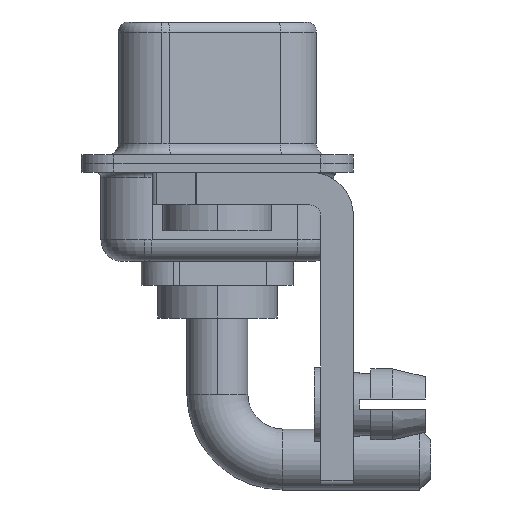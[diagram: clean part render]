
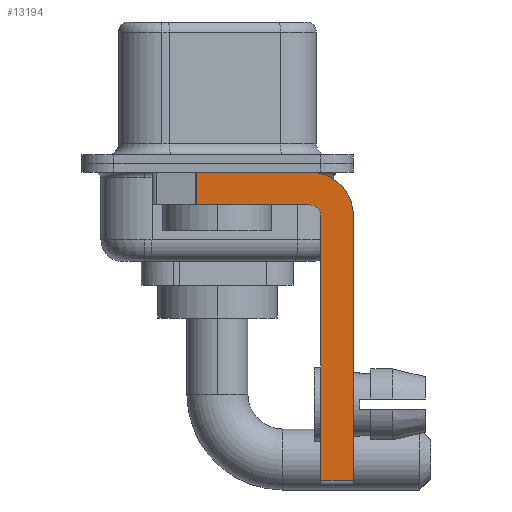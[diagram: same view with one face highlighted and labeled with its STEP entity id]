
A CAD part, left-side view. The second image highlights one B-rep face of the part: STEP entity #13194.
In plain terms, the highlighted planar face has unit normal (-1, 0, 0).
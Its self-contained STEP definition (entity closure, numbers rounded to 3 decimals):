
#27 = EDGE_CURVE ( 'NONE', #10403, #17854, #42, .T. ) ;
#42 = LINE ( 'NONE', #16855, #9133 ) ;
#461 = VECTOR ( 'NONE', #15293, 1000. ) ;
#556 = EDGE_LOOP ( 'NONE', ( #10316, #17344, #16778, #6746, #11287, #14482, #17022, #13312 ) ) ;
#798 = DIRECTION ( 'NONE',  ( 0., 0., -1. ) ) ;
#1170 = CARTESIAN_POINT ( 'NONE',  ( -2.9, 0.978, -1.9 ) ) ;
#2561 = FACE_OUTER_BOUND ( 'NONE', #556, .T. ) ;
#3006 = VERTEX_POINT ( 'NONE', #5183 ) ;
#4519 = CARTESIAN_POINT ( 'NONE',  ( -2.9, -6.25, -2.4 ) ) ;
#4726 = CARTESIAN_POINT ( 'NONE',  ( -2.9, -4.25, -14.55 ) ) ;
#5128 = LINE ( 'NONE', #12518, #461 ) ;
#5183 = CARTESIAN_POINT ( 'NONE',  ( -2.9, 0.978, -0.4 ) ) ;
#5199 = CARTESIAN_POINT ( 'NONE',  ( -2.9, 3., -0.4 ) ) ;
#5729 = LINE ( 'NONE', #5199, #9173 ) ;
#6163 = LINE ( 'NONE', #13279, #12338 ) ;
#6687 = CIRCLE ( 'NONE', #7274, 2. ) ;
#6746 = ORIENTED_EDGE ( 'NONE', *, *, #11887, .F. ) ;
#6772 = CARTESIAN_POINT ( 'NONE',  ( -2.9, -4.75, -14.55 ) ) ;
#7009 = DIRECTION ( 'NONE',  ( 0., 0., -1. ) ) ;
#7118 = VECTOR ( 'NONE', #9987, 1000. ) ;
#7274 = AXIS2_PLACEMENT_3D ( 'NONE', #16981, #11368, #7009 ) ;
#7464 = CARTESIAN_POINT ( 'NONE',  ( -2.9, -4.25, -0.4 ) ) ;
#8281 = VERTEX_POINT ( 'NONE', #7464 ) ;
#9119 = EDGE_CURVE ( 'NONE', #3006, #17854, #5128, .T. ) ;
#9133 = VECTOR ( 'NONE', #17028, 1000. ) ;
#9173 = VECTOR ( 'NONE', #15614, 1000. ) ;
#9432 = VERTEX_POINT ( 'NONE', #6772 ) ;
#9480 = CARTESIAN_POINT ( 'NONE',  ( -2.9, -4.25, -2.4 ) ) ;
#9552 = CARTESIAN_POINT ( 'NONE',  ( -2.9, -4.75, -2.4 ) ) ;
#9987 = DIRECTION ( 'NONE',  ( 0., 0., -1. ) ) ;
#10316 = ORIENTED_EDGE ( 'NONE', *, *, #15480, .F. ) ;
#10332 = DIRECTION ( 'NONE',  ( 0., 0., 1. ) ) ;
#10403 = VERTEX_POINT ( 'NONE', #17775 ) ;
#10493 = VECTOR ( 'NONE', #13405, 1000. ) ;
#10551 = LINE ( 'NONE', #4726, #10493 ) ;
#10670 = EDGE_CURVE ( 'NONE', #9432, #12374, #10551, .T. ) ;
#10712 = CARTESIAN_POINT ( 'NONE',  ( -2.9, -4.25, -2.4 ) ) ;
#11287 = ORIENTED_EDGE ( 'NONE', *, *, #13023, .F. ) ;
#11368 = DIRECTION ( 'NONE',  ( 1., 0., 0. ) ) ;
#11464 = EDGE_CURVE ( 'NONE', #8281, #12178, #6687, .T. ) ;
#11887 = EDGE_CURVE ( 'NONE', #12309, #10403, #14977, .T. ) ;
#12178 = VERTEX_POINT ( 'NONE', #17379 ) ;
#12181 = DIRECTION ( 'NONE',  ( 1., 0., 0. ) ) ;
#12309 = VERTEX_POINT ( 'NONE', #9552 ) ;
#12338 = VECTOR ( 'NONE', #10332, 1000. ) ;
#12374 = VERTEX_POINT ( 'NONE', #16370 ) ;
#12518 = CARTESIAN_POINT ( 'NONE',  ( -2.9, 0.978, -1.9 ) ) ;
#13023 = EDGE_CURVE ( 'NONE', #9432, #12309, #6163, .T. ) ;
#13194 = ADVANCED_FACE ( 'NONE', ( #2561 ), #13463, .F. ) ;
#13279 = CARTESIAN_POINT ( 'NONE',  ( -2.9, -4.75, -14.8 ) ) ;
#13312 = ORIENTED_EDGE ( 'NONE', *, *, #11464, .F. ) ;
#13405 = DIRECTION ( 'NONE',  ( 0., -1., 0. ) ) ;
#13463 = PLANE ( 'NONE',  #17927 ) ;
#13807 = DIRECTION ( 'NONE',  ( 0., 0., 1. ) ) ;
#14321 = LINE ( 'NONE', #4519, #7118 ) ;
#14482 = ORIENTED_EDGE ( 'NONE', *, *, #10670, .T. ) ;
#14977 = CIRCLE ( 'NONE', #15550, 0.5 ) ;
#15119 = DIRECTION ( 'NONE',  ( -1., 0., 0. ) ) ;
#15293 = DIRECTION ( 'NONE',  ( 0., 0., -1. ) ) ;
#15480 = EDGE_CURVE ( 'NONE', #3006, #8281, #5729, .T. ) ;
#15550 = AXIS2_PLACEMENT_3D ( 'NONE', #9480, #15119, #13807 ) ;
#15614 = DIRECTION ( 'NONE',  ( 0., -1., 0. ) ) ;
#16370 = CARTESIAN_POINT ( 'NONE',  ( -2.9, -6.25, -14.55 ) ) ;
#16778 = ORIENTED_EDGE ( 'NONE', *, *, #27, .F. ) ;
#16855 = CARTESIAN_POINT ( 'NONE',  ( -2.9, -4.25, -1.9 ) ) ;
#16981 = CARTESIAN_POINT ( 'NONE',  ( -2.9, -4.25, -2.4 ) ) ;
#17022 = ORIENTED_EDGE ( 'NONE', *, *, #17488, .F. ) ;
#17028 = DIRECTION ( 'NONE',  ( 0., 1., 0. ) ) ;
#17344 = ORIENTED_EDGE ( 'NONE', *, *, #9119, .T. ) ;
#17379 = CARTESIAN_POINT ( 'NONE',  ( -2.9, -6.25, -2.4 ) ) ;
#17488 = EDGE_CURVE ( 'NONE', #12178, #12374, #14321, .T. ) ;
#17775 = CARTESIAN_POINT ( 'NONE',  ( -2.9, -4.25, -1.9 ) ) ;
#17854 = VERTEX_POINT ( 'NONE', #1170 ) ;
#17927 = AXIS2_PLACEMENT_3D ( 'NONE', #10712, #12181, #798 ) ;
